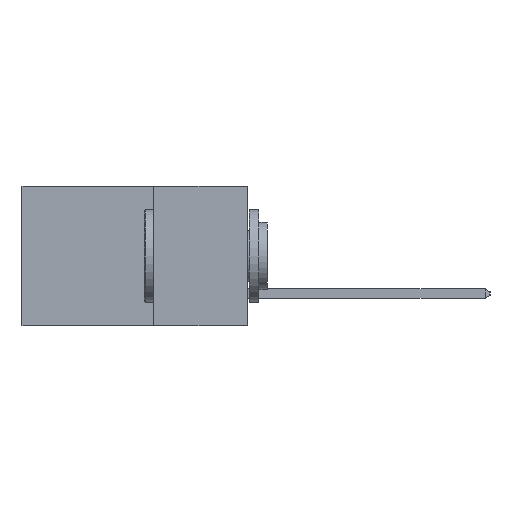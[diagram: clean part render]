
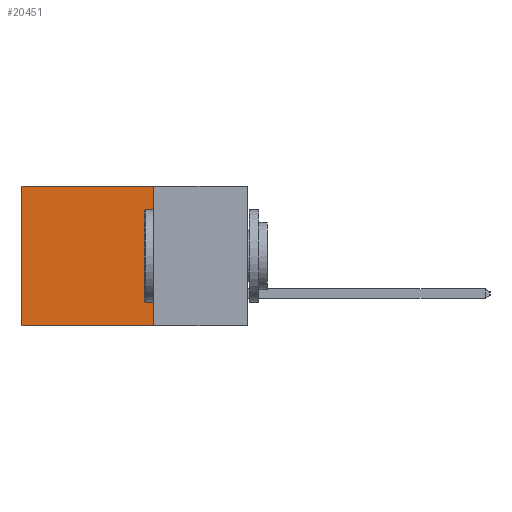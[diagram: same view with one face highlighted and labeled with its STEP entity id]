
A CAD part, left-side view. The second image highlights one B-rep face of the part: STEP entity #20451.
In plain terms, the highlighted planar face has unit normal (-1, 0, 0).
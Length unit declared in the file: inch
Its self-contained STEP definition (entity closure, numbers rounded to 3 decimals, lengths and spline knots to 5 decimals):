
#90 = DIRECTION ( 'NONE',  ( 1., 0., 0. ) ) ;
#727 = VECTOR ( 'NONE', #15908, 39.37008 ) ;
#1877 = VERTEX_POINT ( 'NONE', #7813 ) ;
#2738 = VERTEX_POINT ( 'NONE', #15742 ) ;
#3375 = EDGE_CURVE ( 'NONE', #2738, #9104, #20096, .T. ) ;
#3419 = EDGE_CURVE ( 'NONE', #2738, #1877, #11153, .T. ) ;
#4003 = VERTEX_POINT ( 'NONE', #17668 ) ;
#5979 = ORIENTED_EDGE ( 'NONE', *, *, #3375, .F. ) ;
#7813 = CARTESIAN_POINT ( 'NONE',  ( 0.2615, 0.6, 0. ) ) ;
#8253 = ORIENTED_EDGE ( 'NONE', *, *, #19552, .F. ) ;
#8271 = VECTOR ( 'NONE', #11880, 39.37008 ) ;
#8613 = LINE ( 'NONE', #14309, #727 ) ;
#8980 = EDGE_CURVE ( 'NONE', #1877, #4003, #14151, .T. ) ;
#9104 = VERTEX_POINT ( 'NONE', #10183 ) ;
#9178 = DIRECTION ( 'NONE',  ( 0., 1., 0. ) ) ;
#9229 = CARTESIAN_POINT ( 'NONE',  ( 0.2615, 0.25, 0. ) ) ;
#9793 = DIRECTION ( 'NONE',  ( 0., 0., -1. ) ) ;
#9881 = CARTESIAN_POINT ( 'NONE',  ( 0.2615, 0.25, -0.37 ) ) ;
#10071 = CARTESIAN_POINT ( 'NONE',  ( 0.2615, 0.25, -0.37 ) ) ;
#10183 = CARTESIAN_POINT ( 'NONE',  ( 0.2615, 0.25, -0.37 ) ) ;
#11153 = LINE ( 'NONE', #9229, #14981 ) ;
#11474 = ORIENTED_EDGE ( 'NONE', *, *, #3419, .T. ) ;
#11652 = CARTESIAN_POINT ( 'NONE',  ( 0.2615, 0.6, -0.37 ) ) ;
#11668 = VECTOR ( 'NONE', #9793, 39.37008 ) ;
#11706 = DIRECTION ( 'NONE',  ( 0., 0., -1. ) ) ;
#11858 = AXIS2_PLACEMENT_3D ( 'NONE', #10071, #90, #11706 ) ;
#11880 = DIRECTION ( 'NONE',  ( 0., 0., -1. ) ) ;
#12500 = EDGE_LOOP ( 'NONE', ( #13974, #8253, #5979, #11474 ) ) ;
#13974 = ORIENTED_EDGE ( 'NONE', *, *, #8980, .T. ) ;
#14151 = LINE ( 'NONE', #11652, #8271 ) ;
#14309 = CARTESIAN_POINT ( 'NONE',  ( 0.2615, 0.25, -0.37 ) ) ;
#14981 = VECTOR ( 'NONE', #9178, 39.37008 ) ;
#15742 = CARTESIAN_POINT ( 'NONE',  ( 0.2615, 0.25, 0. ) ) ;
#15908 = DIRECTION ( 'NONE',  ( 0., 1., 0. ) ) ;
#17668 = CARTESIAN_POINT ( 'NONE',  ( 0.2615, 0.6, -0.37 ) ) ;
#19308 = FACE_OUTER_BOUND ( 'NONE', #12500, .T. ) ;
#19552 = EDGE_CURVE ( 'NONE', #9104, #4003, #8613, .T. ) ;
#19604 = PLANE ( 'NONE',  #11858 ) ;
#20096 = LINE ( 'NONE', #9881, #11668 ) ;
#20451 = ADVANCED_FACE ( 'NONE', ( #19308 ), #19604, .F. ) ;
